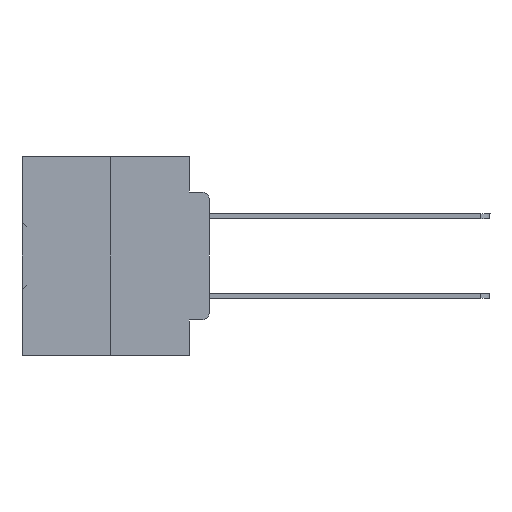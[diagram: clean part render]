
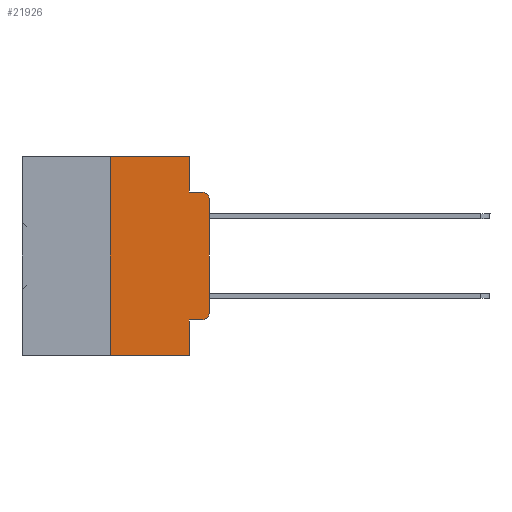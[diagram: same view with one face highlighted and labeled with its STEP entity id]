
A CAD part, left-side view. The second image highlights one B-rep face of the part: STEP entity #21926.
In plain terms, the highlighted planar face has unit normal (-1, 0, 0).
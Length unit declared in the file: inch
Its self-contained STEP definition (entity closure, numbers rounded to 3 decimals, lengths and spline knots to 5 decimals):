
#60 = EDGE_CURVE ( 'NONE', #6252, #22325, #7269, .T. ) ;
#736 = CARTESIAN_POINT ( 'NONE',  ( 0., 0.051, 0. ) ) ;
#992 = CARTESIAN_POINT ( 'NONE',  ( 0., 0.051, -0.0885 ) ) ;
#1525 = CARTESIAN_POINT ( 'NONE',  ( 0., 0.051, -0.4115 ) ) ;
#1553 = VERTEX_POINT ( 'NONE', #29404 ) ;
#2718 = DIRECTION ( 'NONE',  ( 0., 0., 1. ) ) ;
#2966 = CARTESIAN_POINT ( 'NONE',  ( 0., 0.051, -0.5 ) ) ;
#3321 = CIRCLE ( 'NONE', #8226, 0.02 ) ;
#4340 = ORIENTED_EDGE ( 'NONE', *, *, #37886, .F. ) ;
#5356 = EDGE_CURVE ( 'NONE', #11579, #34214, #37178, .T. ) ;
#5908 = LINE ( 'NONE', #6612, #11491 ) ;
#6252 = VERTEX_POINT ( 'NONE', #24386 ) ;
#6299 = LINE ( 'NONE', #736, #36729 ) ;
#6435 = ORIENTED_EDGE ( 'NONE', *, *, #60, .F. ) ;
#6612 = CARTESIAN_POINT ( 'NONE',  ( 0., 0.473, 0. ) ) ;
#7232 = VECTOR ( 'NONE', #30575, 39.37008 ) ;
#7269 = LINE ( 'NONE', #992, #35375 ) ;
#7342 = CARTESIAN_POINT ( 'NONE',  ( 0., 0.25, -0.5 ) ) ;
#7691 = CARTESIAN_POINT ( 'NONE',  ( 0., 0.051, 0. ) ) ;
#7888 = EDGE_CURVE ( 'NONE', #24203, #22325, #3321, .T. ) ;
#8226 = AXIS2_PLACEMENT_3D ( 'NONE', #31347, #16662, #36833 ) ;
#8559 = EDGE_CURVE ( 'NONE', #20163, #1553, #22240, .T. ) ;
#8656 = CARTESIAN_POINT ( 'NONE',  ( 0., 0.051, -0.4115 ) ) ;
#9089 = DIRECTION ( 'NONE',  ( 0., 0., -1. ) ) ;
#9677 = DIRECTION ( 'NONE',  ( 0., -1., 0. ) ) ;
#10389 = LINE ( 'NONE', #18934, #25178 ) ;
#11351 = CARTESIAN_POINT ( 'NONE',  ( 0., 0.25, 0. ) ) ;
#11491 = VECTOR ( 'NONE', #30225, 39.37008 ) ;
#11579 = VERTEX_POINT ( 'NONE', #7342 ) ;
#12099 = EDGE_CURVE ( 'NONE', #32019, #24203, #10389, .T. ) ;
#12967 = ORIENTED_EDGE ( 'NONE', *, *, #7888, .T. ) ;
#13028 = DIRECTION ( 'NONE',  ( -1., 0., 0. ) ) ;
#13569 = ORIENTED_EDGE ( 'NONE', *, *, #8559, .T. ) ;
#13721 = VERTEX_POINT ( 'NONE', #2966 ) ;
#15201 = CIRCLE ( 'NONE', #27609, 0.02 ) ;
#16662 = DIRECTION ( 'NONE',  ( -1., 0., 0. ) ) ;
#17254 = VECTOR ( 'NONE', #22204, 39.37008 ) ;
#17868 = ORIENTED_EDGE ( 'NONE', *, *, #25678, .T. ) ;
#18327 = CARTESIAN_POINT ( 'NONE',  ( 0., 0., -0.3915 ) ) ;
#18784 = CARTESIAN_POINT ( 'NONE',  ( 0., 0.02, -0.0885 ) ) ;
#18863 = ORIENTED_EDGE ( 'NONE', *, *, #25119, .F. ) ;
#18934 = CARTESIAN_POINT ( 'NONE',  ( 0., 0., 0. ) ) ;
#19756 = DIRECTION ( 'NONE',  ( 0., 0., -1. ) ) ;
#19982 = FACE_OUTER_BOUND ( 'NONE', #31502, .T. ) ;
#20163 = VERTEX_POINT ( 'NONE', #1525 ) ;
#20531 = CARTESIAN_POINT ( 'NONE',  ( 0., 0., -0.1085 ) ) ;
#20732 = ORIENTED_EDGE ( 'NONE', *, *, #5356, .F. ) ;
#21643 = DIRECTION ( 'NONE',  ( 0., -1., 0. ) ) ;
#21926 = ADVANCED_FACE ( 'NONE', ( #19982 ), #22968, .F. ) ;
#22204 = DIRECTION ( 'NONE',  ( 0., 0., -1. ) ) ;
#22240 = LINE ( 'NONE', #8656, #27273 ) ;
#22290 = ORIENTED_EDGE ( 'NONE', *, *, #12099, .T. ) ;
#22325 = VERTEX_POINT ( 'NONE', #18784 ) ;
#22968 = PLANE ( 'NONE',  #31358 ) ;
#23229 = DIRECTION ( 'NONE',  ( 1., 0., 0. ) ) ;
#24203 = VERTEX_POINT ( 'NONE', #20531 ) ;
#24283 = CARTESIAN_POINT ( 'NONE',  ( 0., 0.051, 0. ) ) ;
#24386 = CARTESIAN_POINT ( 'NONE',  ( 0., 0.051, -0.0885 ) ) ;
#25119 = EDGE_CURVE ( 'NONE', #34214, #27425, #5908, .T. ) ;
#25178 = VECTOR ( 'NONE', #25265, 39.37008 ) ;
#25265 = DIRECTION ( 'NONE',  ( 0., 0., 1. ) ) ;
#25678 = EDGE_CURVE ( 'NONE', #11579, #13721, #37657, .T. ) ;
#25939 = CARTESIAN_POINT ( 'NONE',  ( 0., 0.473, 0. ) ) ;
#26036 = LINE ( 'NONE', #7691, #17254 ) ;
#27044 = CARTESIAN_POINT ( 'NONE',  ( 0., 0.25, 0. ) ) ;
#27273 = VECTOR ( 'NONE', #9677, 39.37008 ) ;
#27425 = VERTEX_POINT ( 'NONE', #24283 ) ;
#27592 = CARTESIAN_POINT ( 'NONE',  ( 0., 0.02, -0.3915 ) ) ;
#27609 = AXIS2_PLACEMENT_3D ( 'NONE', #27592, #13028, #33135 ) ;
#29404 = CARTESIAN_POINT ( 'NONE',  ( 0., 0.02, -0.4115 ) ) ;
#30148 = EDGE_CURVE ( 'NONE', #1553, #32019, #15201, .T. ) ;
#30225 = DIRECTION ( 'NONE',  ( 0., -1., 0. ) ) ;
#30575 = DIRECTION ( 'NONE',  ( 0., -1., 0. ) ) ;
#31347 = CARTESIAN_POINT ( 'NONE',  ( 0., 0.02, -0.1085 ) ) ;
#31358 = AXIS2_PLACEMENT_3D ( 'NONE', #25939, #23229, #19756 ) ;
#31369 = ORIENTED_EDGE ( 'NONE', *, *, #32616, .F. ) ;
#31502 = EDGE_LOOP ( 'NONE', ( #22290, #12967, #6435, #31369, #18863, #20732, #17868, #4340, #13569, #36511 ) ) ;
#32019 = VERTEX_POINT ( 'NONE', #18327 ) ;
#32616 = EDGE_CURVE ( 'NONE', #27425, #6252, #6299, .T. ) ;
#33135 = DIRECTION ( 'NONE',  ( 0., 0., -1. ) ) ;
#34214 = VERTEX_POINT ( 'NONE', #27044 ) ;
#35375 = VECTOR ( 'NONE', #21643, 39.37008 ) ;
#35754 = VECTOR ( 'NONE', #2718, 39.37008 ) ;
#36083 = CARTESIAN_POINT ( 'NONE',  ( 0., 0.473, -0.5 ) ) ;
#36511 = ORIENTED_EDGE ( 'NONE', *, *, #30148, .T. ) ;
#36729 = VECTOR ( 'NONE', #9089, 39.37008 ) ;
#36833 = DIRECTION ( 'NONE',  ( 0., 0., -1. ) ) ;
#37178 = LINE ( 'NONE', #11351, #35754 ) ;
#37657 = LINE ( 'NONE', #36083, #7232 ) ;
#37886 = EDGE_CURVE ( 'NONE', #20163, #13721, #26036, .T. ) ;
